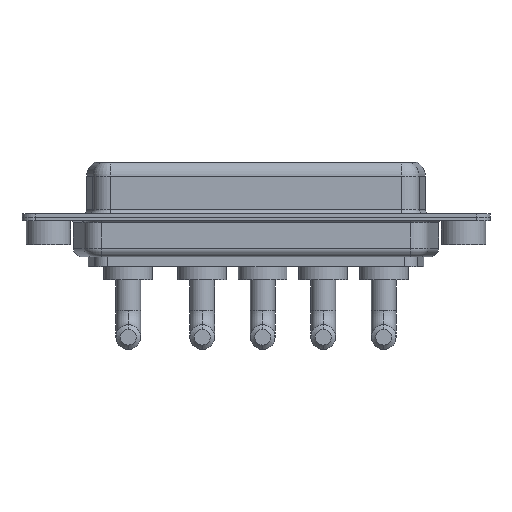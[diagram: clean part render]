
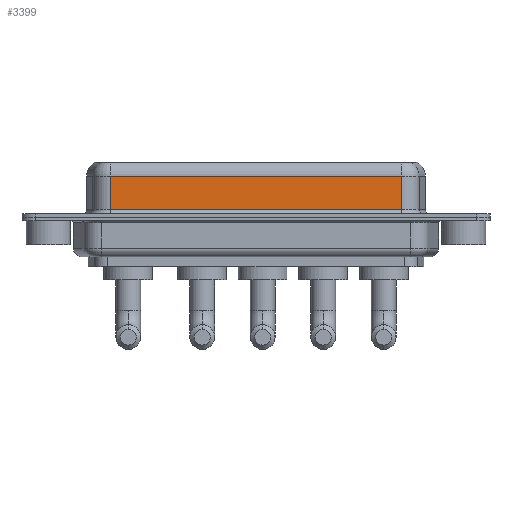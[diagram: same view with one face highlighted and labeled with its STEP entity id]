
A CAD part, front view. The second image highlights one B-rep face of the part: STEP entity #3399.
In plain terms, the highlighted planar face has unit normal (0, -1, 0).
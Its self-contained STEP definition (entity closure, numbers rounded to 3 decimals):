
#127 = VECTOR ( 'NONE', #4684, 1000. ) ;
#233 = DIRECTION ( 'NONE',  ( 0., 1., 0. ) ) ;
#680 = CARTESIAN_POINT ( 'NONE',  ( 7.013, -3.95, 4.65 ) ) ;
#882 = VERTEX_POINT ( 'NONE', #6412 ) ;
#986 = CARTESIAN_POINT ( 'NONE',  ( 40.037, -3.95, 4.65 ) ) ;
#1013 = EDGE_LOOP ( 'NONE', ( #6134, #4344, #11287, #2250 ) ) ;
#1379 = VECTOR ( 'NONE', #7584, 1000. ) ;
#1704 = EDGE_CURVE ( 'NONE', #8457, #3671, #10198, .T. ) ;
#2250 = ORIENTED_EDGE ( 'NONE', *, *, #4343, .T. ) ;
#2818 = CARTESIAN_POINT ( 'NONE',  ( 7.013, -3.95, 6.4 ) ) ;
#3399 = ADVANCED_FACE ( 'NONE', ( #4059 ), #11025, .F. ) ;
#3502 = VERTEX_POINT ( 'NONE', #4304 ) ;
#3671 = VERTEX_POINT ( 'NONE', #680 ) ;
#3690 = LINE ( 'NONE', #11620, #1379 ) ;
#4059 = FACE_OUTER_BOUND ( 'NONE', #1013, .T. ) ;
#4304 = CARTESIAN_POINT ( 'NONE',  ( 40.037, -3.95, 0.9 ) ) ;
#4343 = EDGE_CURVE ( 'NONE', #882, #3502, #11454, .T. ) ;
#4344 = ORIENTED_EDGE ( 'NONE', *, *, #1704, .T. ) ;
#4618 = LINE ( 'NONE', #2818, #127 ) ;
#4684 = DIRECTION ( 'NONE',  ( 0., 0., -1. ) ) ;
#4711 = VECTOR ( 'NONE', #6780, 1000. ) ;
#4890 = AXIS2_PLACEMENT_3D ( 'NONE', #9169, #233, #7880 ) ;
#5206 = DIRECTION ( 'NONE',  ( -1., 0., 0. ) ) ;
#6134 = ORIENTED_EDGE ( 'NONE', *, *, #10746, .F. ) ;
#6412 = CARTESIAN_POINT ( 'NONE',  ( 7.013, -3.95, 0.9 ) ) ;
#6780 = DIRECTION ( 'NONE',  ( 1., 0., 0. ) ) ;
#7584 = DIRECTION ( 'NONE',  ( 0., 0., -1. ) ) ;
#7880 = DIRECTION ( 'NONE',  ( 0., 0., 1. ) ) ;
#8457 = VERTEX_POINT ( 'NONE', #8771 ) ;
#8771 = CARTESIAN_POINT ( 'NONE',  ( 40.037, -3.95, 4.65 ) ) ;
#9169 = CARTESIAN_POINT ( 'NONE',  ( 40.037, -3.95, 6.4 ) ) ;
#9728 = EDGE_CURVE ( 'NONE', #3671, #882, #4618, .T. ) ;
#10198 = LINE ( 'NONE', #986, #11801 ) ;
#10746 = EDGE_CURVE ( 'NONE', #8457, #3502, #3690, .T. ) ;
#11025 = PLANE ( 'NONE',  #4890 ) ;
#11287 = ORIENTED_EDGE ( 'NONE', *, *, #9728, .T. ) ;
#11454 = LINE ( 'NONE', #12663, #4711 ) ;
#11620 = CARTESIAN_POINT ( 'NONE',  ( 40.037, -3.95, 6.4 ) ) ;
#11801 = VECTOR ( 'NONE', #5206, 1000. ) ;
#12663 = CARTESIAN_POINT ( 'NONE',  ( 40.037, -3.95, 0.9 ) ) ;
